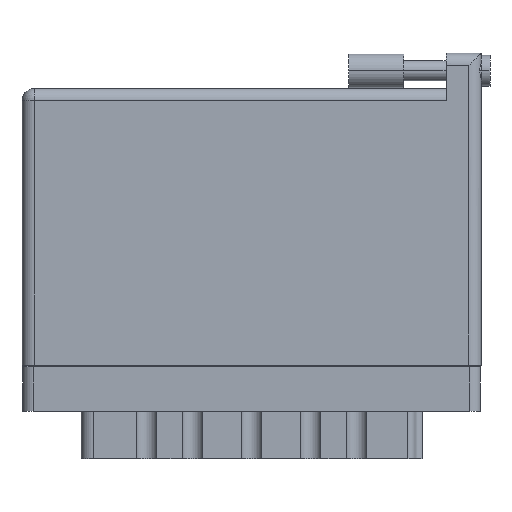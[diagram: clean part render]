
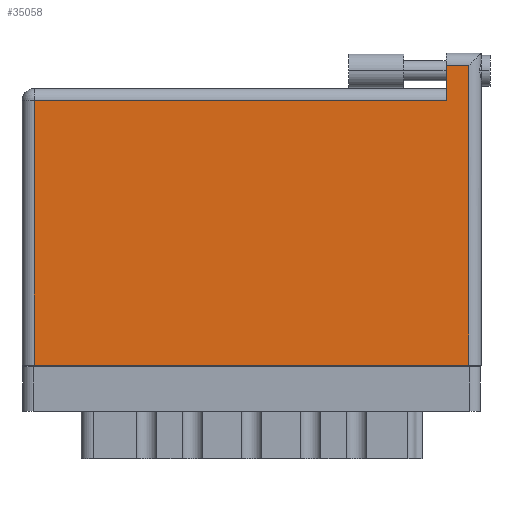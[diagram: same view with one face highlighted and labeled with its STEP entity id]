
A CAD part, front view. The second image highlights one B-rep face of the part: STEP entity #35058.
In plain terms, the highlighted face is planar.
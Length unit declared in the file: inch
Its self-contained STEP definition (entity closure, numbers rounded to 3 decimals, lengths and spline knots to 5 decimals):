
#54 = EDGE_CURVE ( 'NONE', #15680, #6328, #6876, .T. ) ;
#1487 = CARTESIAN_POINT ( 'NONE',  ( 0., 1.696, 0. ) ) ;
#1932 = DIRECTION ( 'NONE',  ( -1., 0., 0. ) ) ;
#2088 = DIRECTION ( 'NONE',  ( 0., 1., 0. ) ) ;
#4982 = CARTESIAN_POINT ( 'NONE',  ( 2.53, 0., 0. ) ) ;
#5677 = FACE_OUTER_BOUND ( 'NONE', #48391, .T. ) ;
#6328 = VERTEX_POINT ( 'NONE', #7437 ) ;
#6876 = LINE ( 'NONE', #22570, #21746 ) ;
#7437 = CARTESIAN_POINT ( 'NONE',  ( 0.07, 0., 0. ) ) ;
#8521 = CARTESIAN_POINT ( 'NONE',  ( 0., 0., 0. ) ) ;
#12348 = LINE ( 'NONE', #16505, #38745 ) ;
#13438 = AXIS2_PLACEMENT_3D ( 'NONE', #51280, #13845, #1932 ) ;
#13845 = DIRECTION ( 'NONE',  ( 0., 0., -1. ) ) ;
#13867 = CARTESIAN_POINT ( 'NONE',  ( 2.403, 1.766, 0. ) ) ;
#14435 = EDGE_CURVE ( 'NONE', #6328, #29763, #43038, .T. ) ;
#15680 = VERTEX_POINT ( 'NONE', #53422 ) ;
#15813 = VERTEX_POINT ( 'NONE', #18818 ) ;
#16505 = CARTESIAN_POINT ( 'NONE',  ( 0., 1.496, 0. ) ) ;
#18818 = CARTESIAN_POINT ( 'NONE',  ( 2.403, 1.696, 0. ) ) ;
#19856 = ORIENTED_EDGE ( 'NONE', *, *, #54, .T. ) ;
#20073 = LINE ( 'NONE', #13867, #47756 ) ;
#21746 = VECTOR ( 'NONE', #43142, 39.37008 ) ;
#22570 = CARTESIAN_POINT ( 'NONE',  ( 0.07, 0., 0. ) ) ;
#22732 = VERTEX_POINT ( 'NONE', #38567 ) ;
#23079 = ORIENTED_EDGE ( 'NONE', *, *, #52850, .T. ) ;
#26851 = LINE ( 'NONE', #51268, #46162 ) ;
#29763 = VERTEX_POINT ( 'NONE', #4982 ) ;
#30434 = DIRECTION ( 'NONE',  ( 0., -1., 0. ) ) ;
#31737 = EDGE_CURVE ( 'NONE', #22732, #15813, #51708, .T. ) ;
#33068 = DIRECTION ( 'NONE',  ( 1., 0., 0. ) ) ;
#34988 = ORIENTED_EDGE ( 'NONE', *, *, #31737, .T. ) ;
#35058 = ADVANCED_FACE ( 'NONE', ( #5677 ), #43050, .F. ) ;
#36337 = VECTOR ( 'NONE', #49443, 39.37008 ) ;
#37440 = DIRECTION ( 'NONE',  ( -1., 0., 0. ) ) ;
#38567 = CARTESIAN_POINT ( 'NONE',  ( 2.53, 1.696, 0. ) ) ;
#38745 = VECTOR ( 'NONE', #37440, 39.37008 ) ;
#38914 = EDGE_CURVE ( 'NONE', #44686, #15680, #12348, .T. ) ;
#42152 = ORIENTED_EDGE ( 'NONE', *, *, #14435, .T. ) ;
#43038 = LINE ( 'NONE', #8521, #48174 ) ;
#43050 = PLANE ( 'NONE',  #13438 ) ;
#43142 = DIRECTION ( 'NONE',  ( 0., -1., 0. ) ) ;
#43280 = ORIENTED_EDGE ( 'NONE', *, *, #38914, .T. ) ;
#44277 = CARTESIAN_POINT ( 'NONE',  ( 2.403, 1.496, 0. ) ) ;
#44686 = VERTEX_POINT ( 'NONE', #44277 ) ;
#45913 = EDGE_CURVE ( 'NONE', #15813, #44686, #20073, .T. ) ;
#46162 = VECTOR ( 'NONE', #2088, 39.37008 ) ;
#47756 = VECTOR ( 'NONE', #30434, 39.37008 ) ;
#48174 = VECTOR ( 'NONE', #33068, 39.37008 ) ;
#48391 = EDGE_LOOP ( 'NONE', ( #42152, #23079, #34988, #53403, #43280, #19856 ) ) ;
#49443 = DIRECTION ( 'NONE',  ( -1., 0., 0. ) ) ;
#51268 = CARTESIAN_POINT ( 'NONE',  ( 2.53, 1.766, 0. ) ) ;
#51280 = CARTESIAN_POINT ( 'NONE',  ( 0., 1.566, 0. ) ) ;
#51708 = LINE ( 'NONE', #1487, #36337 ) ;
#52850 = EDGE_CURVE ( 'NONE', #29763, #22732, #26851, .T. ) ;
#53403 = ORIENTED_EDGE ( 'NONE', *, *, #45913, .T. ) ;
#53422 = CARTESIAN_POINT ( 'NONE',  ( 0.07, 1.496, 0. ) ) ;
